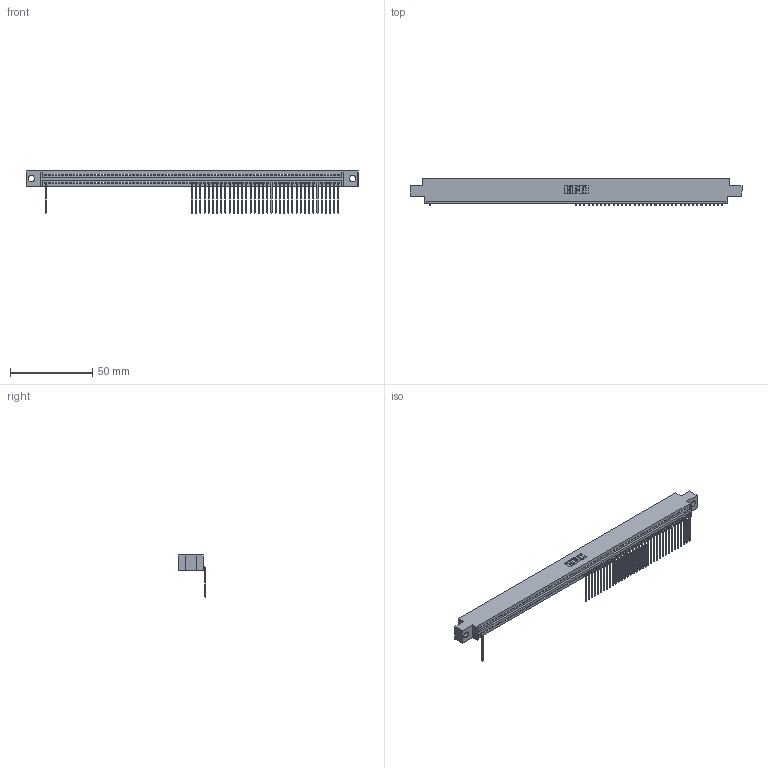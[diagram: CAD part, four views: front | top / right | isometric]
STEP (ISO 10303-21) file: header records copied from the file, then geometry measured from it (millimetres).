
FILE_DESCRIPTION (( 'STEP AP203' ), '1' );
FILE_NAME ('395-071-559-604.STEP', '2018-11-27T07:39:06', ( '' ), ( '' ), 'SwSTEP 2.0', 'SolidWorks 2016', '' );
FILE_SCHEMA (( 'CONFIG_CONTROL_DESIGN' ));
Length unit declared in the file: inch
Products named in the file (3): 345-292-001_558 559 Tail - 1; 395-071-559-604; 345 Part_0.170 Offset - 0.156 Dia-TH
Assembly tree (38 placements, depth 2):
  395-071-559-604
    345 Part_0.170 Offset - 0.156 Dia-TH
    345-292-001_558 559 Tail - 1  x37
Bounding box: 201.55 x 16.75 x 25.53 mm (x, y, z)
Volume: 18913.6 mm3; surface area: 24120.7 mm2
Topology: 38 solids, 38 shells, 2894 faces, 8923 edges, 5898 vertices
Faces by surface type: plane 2114, cylinder 780
Entity records: 48663 total; most frequent: ORIENTED_EDGE 8630, CARTESIAN_POINT 8591, DIRECTION 7421, EDGE_CURVE 4315, VECTOR 3899, LINE 3899, VERTEX_POINT 2874, AXIS2_PLACEMENT_3D 1761
